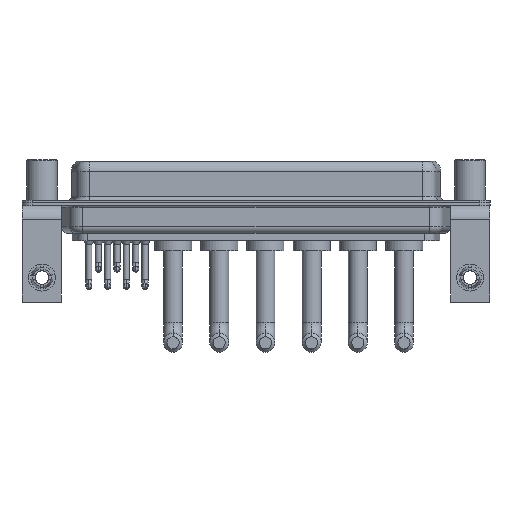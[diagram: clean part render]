
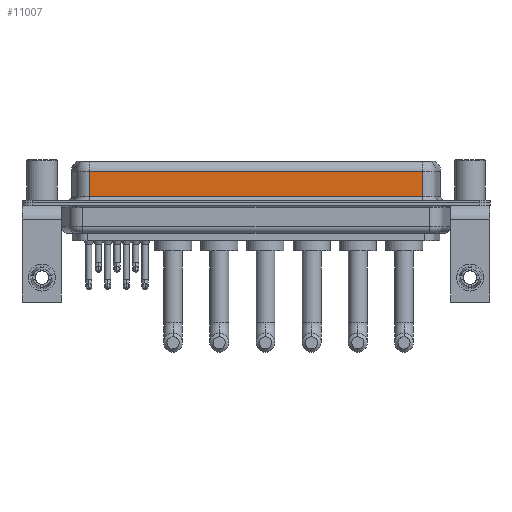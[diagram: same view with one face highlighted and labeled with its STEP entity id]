
A CAD part, front view. The second image highlights one B-rep face of the part: STEP entity #11007.
In plain terms, the highlighted planar face has unit normal (0, -1, 0).
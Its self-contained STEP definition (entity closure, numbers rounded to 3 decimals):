
#252 = VECTOR ( 'NONE', #18790, 1000. ) ;
#536 = CARTESIAN_POINT ( 'NONE',  ( 7.038, -3.95, 6.4 ) ) ;
#744 = LINE ( 'NONE', #21523, #9145 ) ;
#2383 = DIRECTION ( 'NONE',  ( 0., 0., 1. ) ) ;
#2772 = ORIENTED_EDGE ( 'NONE', *, *, #20116, .T. ) ;
#2896 = LINE ( 'NONE', #6430, #252 ) ;
#2898 = EDGE_CURVE ( 'NONE', #10576, #5522, #16180, .T. ) ;
#3066 = EDGE_CURVE ( 'NONE', #3626, #12075, #2896, .T. ) ;
#3626 = VERTEX_POINT ( 'NONE', #12349 ) ;
#4085 = EDGE_LOOP ( 'NONE', ( #21360, #2772, #11653, #15638 ) ) ;
#4474 = CARTESIAN_POINT ( 'NONE',  ( 7.038, -3.95, 4.65 ) ) ;
#5522 = VERTEX_POINT ( 'NONE', #9691 ) ;
#5694 = AXIS2_PLACEMENT_3D ( 'NONE', #7525, #19758, #2383 ) ;
#6430 = CARTESIAN_POINT ( 'NONE',  ( 56.462, -3.95, 6.4 ) ) ;
#7480 = DIRECTION ( 'NONE',  ( 0., 0., -1. ) ) ;
#7525 = CARTESIAN_POINT ( 'NONE',  ( 56.462, -3.95, 6.4 ) ) ;
#8361 = EDGE_CURVE ( 'NONE', #5522, #12075, #744, .T. ) ;
#8966 = VECTOR ( 'NONE', #7480, 1000. ) ;
#9098 = DIRECTION ( 'NONE',  ( -1., 0., 0. ) ) ;
#9145 = VECTOR ( 'NONE', #9750, 1000. ) ;
#9691 = CARTESIAN_POINT ( 'NONE',  ( 7.038, -3.95, 0.9 ) ) ;
#9750 = DIRECTION ( 'NONE',  ( 1., 0., 0. ) ) ;
#10576 = VERTEX_POINT ( 'NONE', #4474 ) ;
#11007 = ADVANCED_FACE ( 'NONE', ( #12784 ), #16223, .F. ) ;
#11653 = ORIENTED_EDGE ( 'NONE', *, *, #2898, .T. ) ;
#12075 = VERTEX_POINT ( 'NONE', #22433 ) ;
#12349 = CARTESIAN_POINT ( 'NONE',  ( 56.462, -3.95, 4.65 ) ) ;
#12784 = FACE_OUTER_BOUND ( 'NONE', #4085, .T. ) ;
#14245 = LINE ( 'NONE', #19162, #14374 ) ;
#14374 = VECTOR ( 'NONE', #9098, 1000. ) ;
#15638 = ORIENTED_EDGE ( 'NONE', *, *, #8361, .T. ) ;
#16180 = LINE ( 'NONE', #536, #8966 ) ;
#16223 = PLANE ( 'NONE',  #5694 ) ;
#18790 = DIRECTION ( 'NONE',  ( 0., 0., -1. ) ) ;
#19162 = CARTESIAN_POINT ( 'NONE',  ( 56.462, -3.95, 4.65 ) ) ;
#19758 = DIRECTION ( 'NONE',  ( 0., 1., 0. ) ) ;
#20116 = EDGE_CURVE ( 'NONE', #3626, #10576, #14245, .T. ) ;
#21360 = ORIENTED_EDGE ( 'NONE', *, *, #3066, .F. ) ;
#21523 = CARTESIAN_POINT ( 'NONE',  ( 56.462, -3.95, 0.9 ) ) ;
#22433 = CARTESIAN_POINT ( 'NONE',  ( 56.462, -3.95, 0.9 ) ) ;
